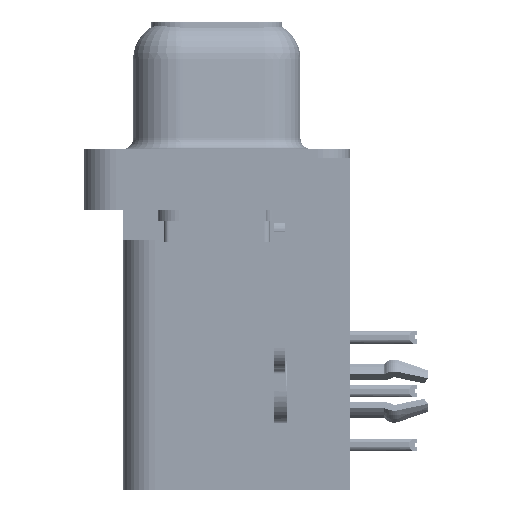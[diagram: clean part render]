
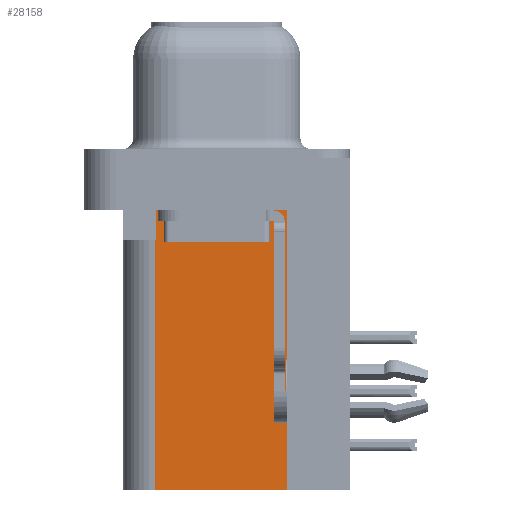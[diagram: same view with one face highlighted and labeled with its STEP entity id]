
A CAD part, left-side view. The second image highlights one B-rep face of the part: STEP entity #28158.
In plain terms, the highlighted planar face has unit normal (-1, 0, 0).
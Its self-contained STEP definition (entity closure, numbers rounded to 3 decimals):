
#2925 = VERTEX_POINT ( 'NONE', #8432 ) ;
#3945 = VECTOR ( 'NONE', #15451, 1000. ) ;
#4432 = ORIENTED_EDGE ( 'NONE', *, *, #8847, .T. ) ;
#4590 = VECTOR ( 'NONE', #14938, 1000. ) ;
#7572 = LINE ( 'NONE', #40701, #52770 ) ;
#8341 = EDGE_CURVE ( 'NONE', #2925, #47856, #23926, .T. ) ;
#8432 = CARTESIAN_POINT ( 'NONE',  ( 3.79, 2.925, -15.7 ) ) ;
#8847 = EDGE_CURVE ( 'NONE', #50515, #21808, #26523, .T. ) ;
#9141 = DIRECTION ( 'NONE',  ( 0., 0., -1. ) ) ;
#9595 = EDGE_CURVE ( 'NONE', #16487, #47856, #18502, .T. ) ;
#10588 = CARTESIAN_POINT ( 'NONE',  ( 3.79, 2.925, -15.7 ) ) ;
#13355 = DIRECTION ( 'NONE',  ( 0., 0., 1. ) ) ;
#13700 = AXIS2_PLACEMENT_3D ( 'NONE', #34425, #34610, #9141 ) ;
#14120 = DIRECTION ( 'NONE',  ( 0., 1., 0. ) ) ;
#14675 = CARTESIAN_POINT ( 'NONE',  ( 3.79, 2.895, -2.5 ) ) ;
#14938 = DIRECTION ( 'NONE',  ( 0., 1., 0. ) ) ;
#15451 = DIRECTION ( 'NONE',  ( 0., 0., -1. ) ) ;
#15818 = ORIENTED_EDGE ( 'NONE', *, *, #8341, .F. ) ;
#16487 = VERTEX_POINT ( 'NONE', #43411 ) ;
#17504 = PLANE ( 'NONE',  #13700 ) ;
#17617 = EDGE_CURVE ( 'NONE', #21808, #49044, #53151, .T. ) ;
#18502 = LINE ( 'NONE', #53017, #4590 ) ;
#20508 = CARTESIAN_POINT ( 'NONE',  ( 3.79, 2.925, -3.9 ) ) ;
#21359 = ORIENTED_EDGE ( 'NONE', *, *, #17617, .T. ) ;
#21808 = VERTEX_POINT ( 'NONE', #25347 ) ;
#22818 = CARTESIAN_POINT ( 'NONE',  ( 3.79, -3.295, -15.7 ) ) ;
#23926 = LINE ( 'NONE', #10588, #47902 ) ;
#25347 = CARTESIAN_POINT ( 'NONE',  ( 3.79, -3.295, -2.5 ) ) ;
#26523 = LINE ( 'NONE', #51572, #49184 ) ;
#28158 = ADVANCED_FACE ( 'NONE', ( #44016 ), #17504, .F. ) ;
#28223 = CARTESIAN_POINT ( 'NONE',  ( 3.79, 2.895, -3.9 ) ) ;
#30988 = EDGE_CURVE ( 'NONE', #49044, #16487, #36506, .T. ) ;
#31496 = ORIENTED_EDGE ( 'NONE', *, *, #34719, .F. ) ;
#32004 = ORIENTED_EDGE ( 'NONE', *, *, #30988, .T. ) ;
#34425 = CARTESIAN_POINT ( 'NONE',  ( 3.79, -3.295, -15.7 ) ) ;
#34610 = DIRECTION ( 'NONE',  ( 1., 0., 0. ) ) ;
#34719 = EDGE_CURVE ( 'NONE', #50515, #2925, #7572, .T. ) ;
#36506 = LINE ( 'NONE', #28223, #3945 ) ;
#40300 = DIRECTION ( 'NONE',  ( 0., 0., 1. ) ) ;
#40701 = CARTESIAN_POINT ( 'NONE',  ( 3.79, -3.295, -15.7 ) ) ;
#43411 = CARTESIAN_POINT ( 'NONE',  ( 3.79, 2.895, -3.9 ) ) ;
#43845 = CARTESIAN_POINT ( 'NONE',  ( 3.79, -3.295, -2.5 ) ) ;
#44016 = FACE_OUTER_BOUND ( 'NONE', #52852, .T. ) ;
#44794 = DIRECTION ( 'NONE',  ( 0., 1., 0. ) ) ;
#45824 = ORIENTED_EDGE ( 'NONE', *, *, #9595, .T. ) ;
#47856 = VERTEX_POINT ( 'NONE', #20508 ) ;
#47902 = VECTOR ( 'NONE', #40300, 1000. ) ;
#49044 = VERTEX_POINT ( 'NONE', #14675 ) ;
#49184 = VECTOR ( 'NONE', #13355, 1000. ) ;
#50515 = VERTEX_POINT ( 'NONE', #22818 ) ;
#51572 = CARTESIAN_POINT ( 'NONE',  ( 3.79, -3.295, -15.7 ) ) ;
#51794 = VECTOR ( 'NONE', #14120, 1000. ) ;
#52770 = VECTOR ( 'NONE', #44794, 1000. ) ;
#52852 = EDGE_LOOP ( 'NONE', ( #21359, #32004, #45824, #15818, #31496, #4432 ) ) ;
#53017 = CARTESIAN_POINT ( 'NONE',  ( 3.79, 0., -3.9 ) ) ;
#53151 = LINE ( 'NONE', #43845, #51794 ) ;
